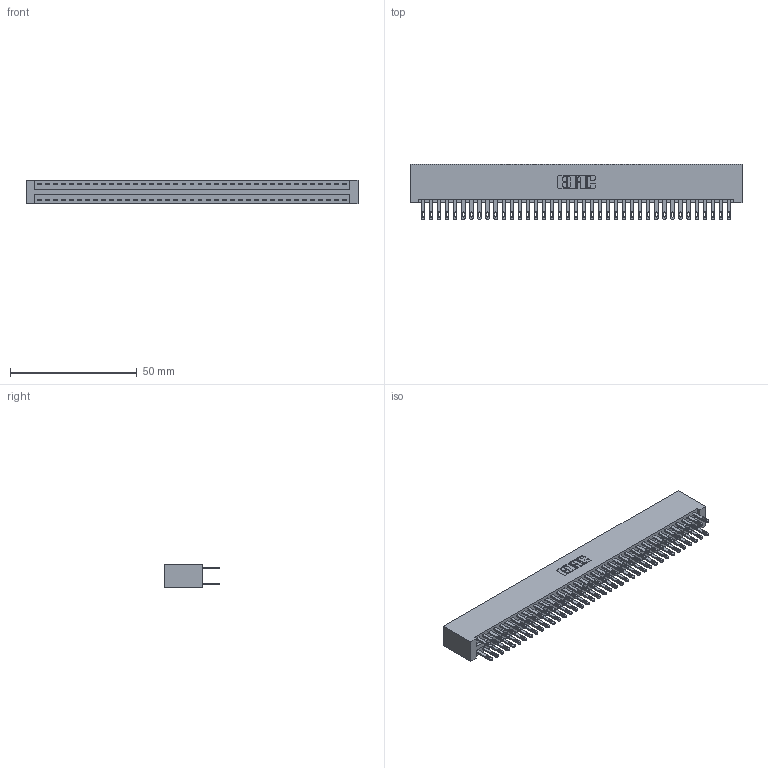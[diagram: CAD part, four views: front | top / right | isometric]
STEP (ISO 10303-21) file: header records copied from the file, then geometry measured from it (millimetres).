
FILE_DESCRIPTION (( 'STEP AP203' ), '1' );
FILE_NAME ('346-078-500-201.STEP', '2022-05-25T13:21:26', ( '' ), ( '' ), 'SwSTEP 2.0', 'SolidWorks 2020', '' );
FILE_SCHEMA (( 'CONFIG_CONTROL_DESIGN' ));
Length unit declared in the file: inch
Products named in the file (3): 346-078-500-201; 346 Part_No Mounting Lugs; 345-292-001_345-293-100
Assembly tree (79 placements, depth 2):
  346-078-500-201
    346 Part_No Mounting Lugs
    345-292-001_345-293-100  x78
Bounding box: 131.06 x 21.84 x 9.4 mm (x, y, z)
Volume: 13568.7 mm3; surface area: 19583.5 mm2
Topology: 79 solids, 79 shells, 3858 faces, 11771 edges, 7846 vertices
Faces by surface type: plane 2334, cylinder 1524
Entity records: 25509 total; most frequent: CARTESIAN_POINT 4204, ORIENTED_EDGE 4138, DIRECTION 3753, EDGE_CURVE 2069, VECTOR 1785, LINE 1785, VERTEX_POINT 1378, AXIS2_PLACEMENT_3D 984
